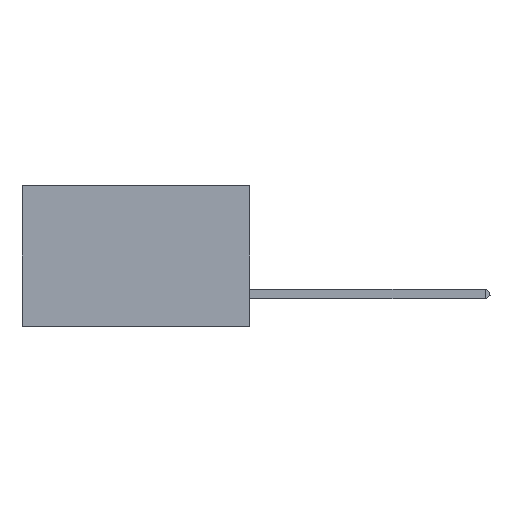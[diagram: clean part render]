
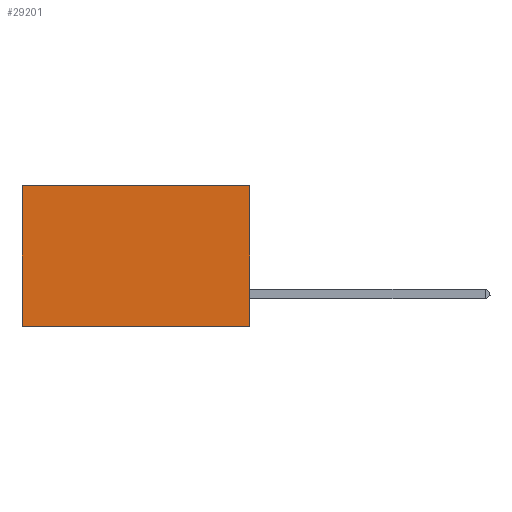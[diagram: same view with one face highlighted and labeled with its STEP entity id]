
A CAD part, left-side view. The second image highlights one B-rep face of the part: STEP entity #29201.
In plain terms, the highlighted planar face has unit normal (-1, 0, 0).
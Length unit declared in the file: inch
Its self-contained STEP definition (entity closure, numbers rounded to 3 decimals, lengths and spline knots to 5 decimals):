
#211 = CARTESIAN_POINT ( 'NONE',  ( 0.2875, 0., 0. ) ) ;
#761 = LINE ( 'NONE', #34501, #16766 ) ;
#1111 = CARTESIAN_POINT ( 'NONE',  ( 0.2875, 0.6, -0.37 ) ) ;
#1192 = LINE ( 'NONE', #45460, #26993 ) ;
#2180 = PLANE ( 'NONE',  #15939 ) ;
#5284 = CARTESIAN_POINT ( 'NONE',  ( 0.2875, 0.6, 0. ) ) ;
#5316 = CARTESIAN_POINT ( 'NONE',  ( 0.2875, 0., -0.37 ) ) ;
#6365 = VERTEX_POINT ( 'NONE', #5284 ) ;
#7552 = DIRECTION ( 'NONE',  ( 0., 1., 0. ) ) ;
#7970 = CARTESIAN_POINT ( 'NONE',  ( 0.2875, 0.6, 0. ) ) ;
#9286 = VERTEX_POINT ( 'NONE', #1111 ) ;
#10165 = CARTESIAN_POINT ( 'NONE',  ( 0.2875, 0., 0. ) ) ;
#10297 = LINE ( 'NONE', #7970, #24052 ) ;
#11067 = EDGE_CURVE ( 'NONE', #22042, #33819, #761, .T. ) ;
#11662 = DIRECTION ( 'NONE',  ( 0., 0., -1. ) ) ;
#15939 = AXIS2_PLACEMENT_3D ( 'NONE', #27809, #30838, #38351 ) ;
#16021 = EDGE_CURVE ( 'NONE', #6365, #9286, #10297, .T. ) ;
#16766 = VECTOR ( 'NONE', #27485, 39.37008 ) ;
#19051 = EDGE_LOOP ( 'NONE', ( #25796, #45997, #34747, #35729 ) ) ;
#22042 = VERTEX_POINT ( 'NONE', #10165 ) ;
#24052 = VECTOR ( 'NONE', #11662, 39.37008 ) ;
#25796 = ORIENTED_EDGE ( 'NONE', *, *, #16021, .T. ) ;
#26000 = VECTOR ( 'NONE', #7552, 39.37008 ) ;
#26993 = VECTOR ( 'NONE', #38105, 39.37008 ) ;
#27485 = DIRECTION ( 'NONE',  ( 0., 0., -1. ) ) ;
#27809 = CARTESIAN_POINT ( 'NONE',  ( 0.2875, 0., 0. ) ) ;
#28331 = EDGE_CURVE ( 'NONE', #22042, #6365, #39117, .T. ) ;
#29201 = ADVANCED_FACE ( 'NONE', ( #38428 ), #2180, .F. ) ;
#30838 = DIRECTION ( 'NONE',  ( 1., 0., 0. ) ) ;
#33819 = VERTEX_POINT ( 'NONE', #5316 ) ;
#34501 = CARTESIAN_POINT ( 'NONE',  ( 0.2875, 0., 0. ) ) ;
#34747 = ORIENTED_EDGE ( 'NONE', *, *, #11067, .F. ) ;
#35729 = ORIENTED_EDGE ( 'NONE', *, *, #28331, .T. ) ;
#38105 = DIRECTION ( 'NONE',  ( 0., 1., 0. ) ) ;
#38351 = DIRECTION ( 'NONE',  ( 0., 0., -1. ) ) ;
#38428 = FACE_OUTER_BOUND ( 'NONE', #19051, .T. ) ;
#39117 = LINE ( 'NONE', #211, #26000 ) ;
#45388 = EDGE_CURVE ( 'NONE', #33819, #9286, #1192, .T. ) ;
#45460 = CARTESIAN_POINT ( 'NONE',  ( 0.2875, 0., -0.37 ) ) ;
#45997 = ORIENTED_EDGE ( 'NONE', *, *, #45388, .F. ) ;
